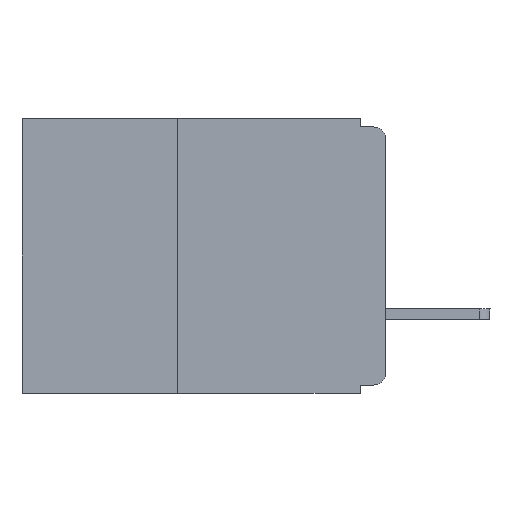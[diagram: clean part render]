
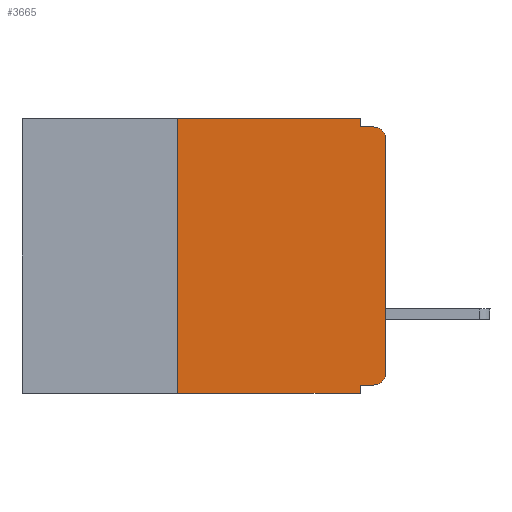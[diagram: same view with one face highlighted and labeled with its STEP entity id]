
A CAD part, left-side view. The second image highlights one B-rep face of the part: STEP entity #3665.
In plain terms, the highlighted planar face has unit normal (-1, 0, 0).
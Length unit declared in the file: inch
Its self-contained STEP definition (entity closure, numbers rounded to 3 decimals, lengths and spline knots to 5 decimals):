
#8 = VECTOR ( 'NONE', #15290, 39.37008 ) ;
#144 = LINE ( 'NONE', #4621, #564 ) ;
#165 = VERTEX_POINT ( 'NONE', #5508 ) ;
#404 = ORIENTED_EDGE ( 'NONE', *, *, #13412, .T. ) ;
#458 = LINE ( 'NONE', #16539, #12512 ) ;
#564 = VECTOR ( 'NONE', #11379, 39.37008 ) ;
#591 = DIRECTION ( 'NONE',  ( 0., 0., 1. ) ) ;
#853 = CARTESIAN_POINT ( 'NONE',  ( 0., 0.015, -0.32 ) ) ;
#950 = EDGE_CURVE ( 'NONE', #4882, #13332, #8935, .T. ) ;
#1140 = EDGE_CURVE ( 'NONE', #2367, #4446, #4153, .T. ) ;
#1203 = CARTESIAN_POINT ( 'NONE',  ( 0., 0., -0.32 ) ) ;
#1733 = VERTEX_POINT ( 'NONE', #15308 ) ;
#1812 = CARTESIAN_POINT ( 'NONE',  ( 0., 0.437, 0. ) ) ;
#2286 = VECTOR ( 'NONE', #7014, 39.37008 ) ;
#2367 = VERTEX_POINT ( 'NONE', #853 ) ;
#2538 = EDGE_CURVE ( 'NONE', #14648, #165, #16004, .T. ) ;
#2974 = PLANE ( 'NONE',  #4083 ) ;
#3665 = ADVANCED_FACE ( 'NONE', ( #12211 ), #2974, .F. ) ;
#3901 = EDGE_CURVE ( 'NONE', #1733, #6256, #144, .T. ) ;
#4058 = EDGE_LOOP ( 'NONE', ( #16420, #404, #11021, #7759, #6278, #13428, #7491, #11648, #5709, #7562 ) ) ;
#4083 = AXIS2_PLACEMENT_3D ( 'NONE', #5465, #9511, #5345 ) ;
#4134 = CARTESIAN_POINT ( 'NONE',  ( 0., 0.015, -0.305 ) ) ;
#4153 = LINE ( 'NONE', #1203, #12487 ) ;
#4165 = LINE ( 'NONE', #5454, #14746 ) ;
#4282 = LINE ( 'NONE', #5114, #14459 ) ;
#4446 = VERTEX_POINT ( 'NONE', #11200 ) ;
#4621 = CARTESIAN_POINT ( 'NONE',  ( 0., 0., -0.01 ) ) ;
#4882 = VERTEX_POINT ( 'NONE', #10776 ) ;
#5114 = CARTESIAN_POINT ( 'NONE',  ( 0., 0.031, -0.33 ) ) ;
#5345 = DIRECTION ( 'NONE',  ( 0., 0., -1. ) ) ;
#5454 = CARTESIAN_POINT ( 'NONE',  ( 0., 0., 0. ) ) ;
#5465 = CARTESIAN_POINT ( 'NONE',  ( 0., 0.437, 0. ) ) ;
#5508 = CARTESIAN_POINT ( 'NONE',  ( 0., 0.031, 0. ) ) ;
#5620 = DIRECTION ( 'NONE',  ( 0., 0., -1. ) ) ;
#5709 = ORIENTED_EDGE ( 'NONE', *, *, #1140, .F. ) ;
#6256 = VERTEX_POINT ( 'NONE', #7640 ) ;
#6278 = ORIENTED_EDGE ( 'NONE', *, *, #2538, .F. ) ;
#6792 = VERTEX_POINT ( 'NONE', #14164 ) ;
#7014 = DIRECTION ( 'NONE',  ( 0., -1., 0. ) ) ;
#7491 = ORIENTED_EDGE ( 'NONE', *, *, #950, .T. ) ;
#7562 = ORIENTED_EDGE ( 'NONE', *, *, #9151, .T. ) ;
#7623 = CARTESIAN_POINT ( 'NONE',  ( 0., 0., -0.025 ) ) ;
#7640 = CARTESIAN_POINT ( 'NONE',  ( 0., 0.015, -0.01 ) ) ;
#7759 = ORIENTED_EDGE ( 'NONE', *, *, #12372, .F. ) ;
#7874 = CARTESIAN_POINT ( 'NONE',  ( 0., 0.015, -0.025 ) ) ;
#8013 = DIRECTION ( 'NONE',  ( 0., 0., -1. ) ) ;
#8270 = DIRECTION ( 'NONE',  ( -1., 0., 0. ) ) ;
#8867 = CIRCLE ( 'NONE', #12471, 0.015 ) ;
#8935 = LINE ( 'NONE', #16572, #12922 ) ;
#9034 = CARTESIAN_POINT ( 'NONE',  ( 0., 0.031, -0.33 ) ) ;
#9151 = EDGE_CURVE ( 'NONE', #2367, #6792, #12371, .T. ) ;
#9511 = DIRECTION ( 'NONE',  ( 1., 0., 0. ) ) ;
#9828 = VERTEX_POINT ( 'NONE', #7623 ) ;
#10040 = CARTESIAN_POINT ( 'NONE',  ( 0., 0.031, 0. ) ) ;
#10776 = CARTESIAN_POINT ( 'NONE',  ( 0., 0.25, -0.33 ) ) ;
#11021 = ORIENTED_EDGE ( 'NONE', *, *, #3901, .F. ) ;
#11170 = DIRECTION ( 'NONE',  ( 0., -1., 0. ) ) ;
#11200 = CARTESIAN_POINT ( 'NONE',  ( 0., 0.031, -0.32 ) ) ;
#11379 = DIRECTION ( 'NONE',  ( 0., -1., 0. ) ) ;
#11607 = CARTESIAN_POINT ( 'NONE',  ( 0., 0.25, 0. ) ) ;
#11626 = EDGE_CURVE ( 'NONE', #4882, #14648, #458, .T. ) ;
#11648 = ORIENTED_EDGE ( 'NONE', *, *, #14348, .F. ) ;
#11713 = DIRECTION ( 'NONE',  ( 0., 0., -1. ) ) ;
#12211 = FACE_OUTER_BOUND ( 'NONE', #4058, .T. ) ;
#12371 = CIRCLE ( 'NONE', #13783, 0.015 ) ;
#12372 = EDGE_CURVE ( 'NONE', #165, #1733, #16413, .T. ) ;
#12471 = AXIS2_PLACEMENT_3D ( 'NONE', #7874, #8270, #5620 ) ;
#12487 = VECTOR ( 'NONE', #13097, 39.37008 ) ;
#12512 = VECTOR ( 'NONE', #13686, 39.37008 ) ;
#12922 = VECTOR ( 'NONE', #11170, 39.37008 ) ;
#13097 = DIRECTION ( 'NONE',  ( 0., 1., 0. ) ) ;
#13332 = VERTEX_POINT ( 'NONE', #9034 ) ;
#13412 = EDGE_CURVE ( 'NONE', #9828, #6256, #8867, .T. ) ;
#13428 = ORIENTED_EDGE ( 'NONE', *, *, #11626, .F. ) ;
#13686 = DIRECTION ( 'NONE',  ( 0., 0., 1. ) ) ;
#13783 = AXIS2_PLACEMENT_3D ( 'NONE', #4134, #14586, #8013 ) ;
#14164 = CARTESIAN_POINT ( 'NONE',  ( 0., 0., -0.305 ) ) ;
#14348 = EDGE_CURVE ( 'NONE', #4446, #13332, #4282, .T. ) ;
#14459 = VECTOR ( 'NONE', #11713, 39.37008 ) ;
#14586 = DIRECTION ( 'NONE',  ( -1., 0., 0. ) ) ;
#14648 = VERTEX_POINT ( 'NONE', #11607 ) ;
#14746 = VECTOR ( 'NONE', #591, 39.37008 ) ;
#15290 = DIRECTION ( 'NONE',  ( 0., 0., -1. ) ) ;
#15308 = CARTESIAN_POINT ( 'NONE',  ( 0., 0.031, -0.01 ) ) ;
#16004 = LINE ( 'NONE', #1812, #2286 ) ;
#16047 = EDGE_CURVE ( 'NONE', #6792, #9828, #4165, .T. ) ;
#16413 = LINE ( 'NONE', #10040, #8 ) ;
#16420 = ORIENTED_EDGE ( 'NONE', *, *, #16047, .T. ) ;
#16539 = CARTESIAN_POINT ( 'NONE',  ( 0., 0.25, -0.33 ) ) ;
#16572 = CARTESIAN_POINT ( 'NONE',  ( 0., 0.437, -0.33 ) ) ;
